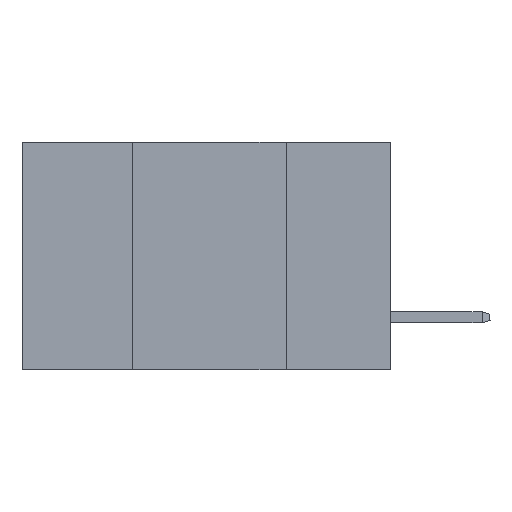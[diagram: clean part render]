
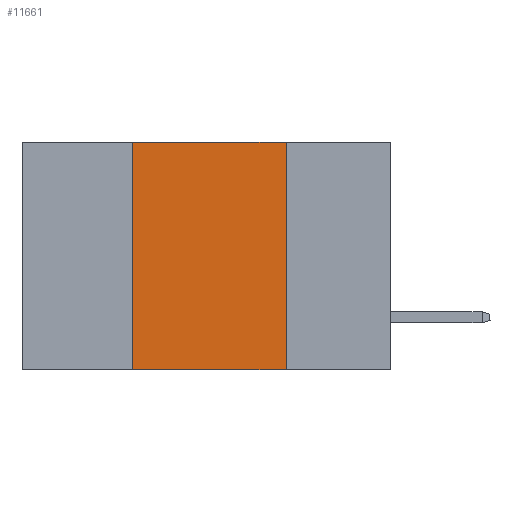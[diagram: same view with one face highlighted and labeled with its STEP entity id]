
A CAD part, left-side view. The second image highlights one B-rep face of the part: STEP entity #11661.
In plain terms, the highlighted planar face has unit normal (-1, 0, 0).
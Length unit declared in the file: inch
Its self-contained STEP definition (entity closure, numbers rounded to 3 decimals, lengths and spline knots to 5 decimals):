
#76 = CARTESIAN_POINT ( 'NONE',  ( 0., 0.17, -0.37 ) ) ;
#223 = AXIS2_PLACEMENT_3D ( 'NONE', #975, #5825, #14683 ) ;
#660 = EDGE_CURVE ( 'NONE', #1215, #9881, #3490, .T. ) ;
#975 = CARTESIAN_POINT ( 'NONE',  ( 0., 0.6, 0. ) ) ;
#1215 = VERTEX_POINT ( 'NONE', #4255 ) ;
#1338 = FACE_OUTER_BOUND ( 'NONE', #6153, .T. ) ;
#2471 = ORIENTED_EDGE ( 'NONE', *, *, #13208, .F. ) ;
#3490 = LINE ( 'NONE', #10851, #13109 ) ;
#3710 = DIRECTION ( 'NONE',  ( 0., -1., 0. ) ) ;
#4255 = CARTESIAN_POINT ( 'NONE',  ( 0., 0.42, -0.37 ) ) ;
#4404 = VECTOR ( 'NONE', #3710, 39.37008 ) ;
#5068 = VERTEX_POINT ( 'NONE', #11379 ) ;
#5188 = CARTESIAN_POINT ( 'NONE',  ( 0., 0.6, 0. ) ) ;
#5453 = ORIENTED_EDGE ( 'NONE', *, *, #660, .F. ) ;
#5825 = DIRECTION ( 'NONE',  ( 1., 0., 0. ) ) ;
#6153 = EDGE_LOOP ( 'NONE', ( #15807, #2471, #5453, #8949 ) ) ;
#7069 = PLANE ( 'NONE',  #223 ) ;
#7687 = EDGE_CURVE ( 'NONE', #5068, #10860, #11127, .T. ) ;
#8745 = VECTOR ( 'NONE', #14006, 39.37008 ) ;
#8949 = ORIENTED_EDGE ( 'NONE', *, *, #15542, .T. ) ;
#9135 = LINE ( 'NONE', #5188, #8745 ) ;
#9526 = DIRECTION ( 'NONE',  ( 0., 0., -1. ) ) ;
#9881 = VERTEX_POINT ( 'NONE', #14136 ) ;
#10644 = CARTESIAN_POINT ( 'NONE',  ( 0., 0.17, 0. ) ) ;
#10803 = DIRECTION ( 'NONE',  ( 0., 0., 1. ) ) ;
#10851 = CARTESIAN_POINT ( 'NONE',  ( 0., 0.42, 0. ) ) ;
#10860 = VERTEX_POINT ( 'NONE', #76 ) ;
#11127 = LINE ( 'NONE', #10644, #12711 ) ;
#11379 = CARTESIAN_POINT ( 'NONE',  ( 0., 0.17, 0. ) ) ;
#11661 = ADVANCED_FACE ( 'NONE', ( #1338 ), #7069, .F. ) ;
#12694 = LINE ( 'NONE', #13697, #4404 ) ;
#12711 = VECTOR ( 'NONE', #9526, 39.37008 ) ;
#13109 = VECTOR ( 'NONE', #10803, 39.37008 ) ;
#13208 = EDGE_CURVE ( 'NONE', #9881, #5068, #9135, .T. ) ;
#13697 = CARTESIAN_POINT ( 'NONE',  ( 0., 0.6, -0.37 ) ) ;
#14006 = DIRECTION ( 'NONE',  ( 0., -1., 0. ) ) ;
#14136 = CARTESIAN_POINT ( 'NONE',  ( 0., 0.42, 0. ) ) ;
#14683 = DIRECTION ( 'NONE',  ( 0., 0., -1. ) ) ;
#15542 = EDGE_CURVE ( 'NONE', #1215, #10860, #12694, .T. ) ;
#15807 = ORIENTED_EDGE ( 'NONE', *, *, #7687, .F. ) ;
